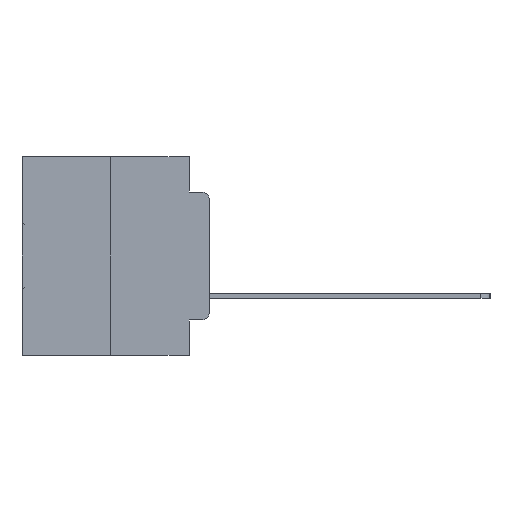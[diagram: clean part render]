
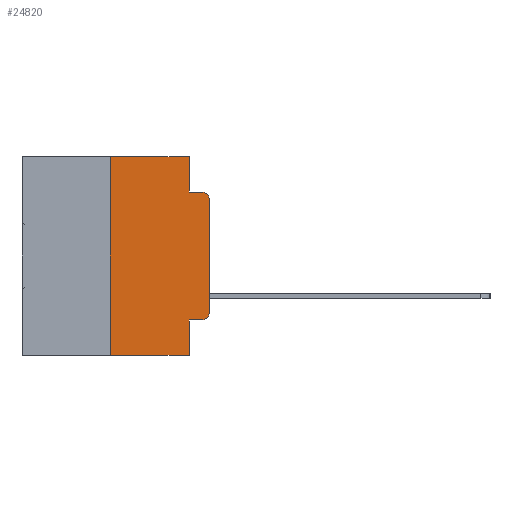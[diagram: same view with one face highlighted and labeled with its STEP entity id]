
A CAD part, left-side view. The second image highlights one B-rep face of the part: STEP entity #24820.
In plain terms, the highlighted planar face has unit normal (-1, 0, 0).
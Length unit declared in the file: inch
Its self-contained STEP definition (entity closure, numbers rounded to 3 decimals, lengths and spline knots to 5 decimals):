
#988 = VERTEX_POINT ( 'NONE', #23663 ) ;
#1040 = CARTESIAN_POINT ( 'NONE',  ( 0., 0.02, -0.3915 ) ) ;
#1591 = EDGE_CURVE ( 'NONE', #27273, #22141, #10794, .T. ) ;
#3335 = CARTESIAN_POINT ( 'NONE',  ( 0., 0., 0. ) ) ;
#3458 = ORIENTED_EDGE ( 'NONE', *, *, #25000, .T. ) ;
#3571 = DIRECTION ( 'NONE',  ( 0., 0., -1. ) ) ;
#3764 = VERTEX_POINT ( 'NONE', #28534 ) ;
#4169 = DIRECTION ( 'NONE',  ( 0., 0., 1. ) ) ;
#4621 = VERTEX_POINT ( 'NONE', #22576 ) ;
#4891 = AXIS2_PLACEMENT_3D ( 'NONE', #10089, #24775, #10200 ) ;
#5931 = LINE ( 'NONE', #25478, #31104 ) ;
#6651 = CARTESIAN_POINT ( 'NONE',  ( 0., 0.02, -0.1085 ) ) ;
#6950 = CARTESIAN_POINT ( 'NONE',  ( 0., 0.051, -0.4115 ) ) ;
#6999 = ORIENTED_EDGE ( 'NONE', *, *, #1591, .F. ) ;
#7049 = FACE_OUTER_BOUND ( 'NONE', #20201, .T. ) ;
#7305 = CARTESIAN_POINT ( 'NONE',  ( 0., 0.051, 0. ) ) ;
#7730 = PLANE ( 'NONE',  #4891 ) ;
#8186 = ORIENTED_EDGE ( 'NONE', *, *, #10568, .F. ) ;
#8325 = CARTESIAN_POINT ( 'NONE',  ( 0., 0.051, -0.4115 ) ) ;
#8452 = DIRECTION ( 'NONE',  ( 0., -1., 0. ) ) ;
#9172 = DIRECTION ( 'NONE',  ( 0., 0., -1. ) ) ;
#9244 = AXIS2_PLACEMENT_3D ( 'NONE', #1040, #18302, #3571 ) ;
#10089 = CARTESIAN_POINT ( 'NONE',  ( 0., 0.473, 0. ) ) ;
#10200 = DIRECTION ( 'NONE',  ( 0., 0., -1. ) ) ;
#10288 = VERTEX_POINT ( 'NONE', #20030 ) ;
#10474 = EDGE_CURVE ( 'NONE', #10288, #25255, #24350, .T. ) ;
#10568 = EDGE_CURVE ( 'NONE', #11754, #3764, #27742, .T. ) ;
#10794 = LINE ( 'NONE', #30695, #17292 ) ;
#11110 = EDGE_CURVE ( 'NONE', #22141, #13493, #5931, .T. ) ;
#11323 = EDGE_CURVE ( 'NONE', #20082, #27273, #25884, .T. ) ;
#11754 = VERTEX_POINT ( 'NONE', #8325 ) ;
#11922 = CARTESIAN_POINT ( 'NONE',  ( 0., 0.473, -0.5 ) ) ;
#12048 = EDGE_CURVE ( 'NONE', #4621, #3764, #23223, .T. ) ;
#12627 = CARTESIAN_POINT ( 'NONE',  ( 0., 0.051, -0.0885 ) ) ;
#13260 = DIRECTION ( 'NONE',  ( 0., 0., 1. ) ) ;
#13493 = VERTEX_POINT ( 'NONE', #22747 ) ;
#13698 = CARTESIAN_POINT ( 'NONE',  ( 0., 0.051, 0. ) ) ;
#13755 = EDGE_CURVE ( 'NONE', #4621, #20082, #24603, .T. ) ;
#14351 = DIRECTION ( 'NONE',  ( 0., -1., 0. ) ) ;
#14838 = VECTOR ( 'NONE', #25820, 39.37008 ) ;
#15492 = VECTOR ( 'NONE', #13260, 39.37008 ) ;
#16269 = LINE ( 'NONE', #3335, #15492 ) ;
#16579 = CARTESIAN_POINT ( 'NONE',  ( 0., 0.473, 0. ) ) ;
#17292 = VECTOR ( 'NONE', #28388, 39.37008 ) ;
#17509 = VECTOR ( 'NONE', #28945, 39.37008 ) ;
#17864 = VECTOR ( 'NONE', #14351, 39.37008 ) ;
#18302 = DIRECTION ( 'NONE',  ( -1., 0., 0. ) ) ;
#18519 = ORIENTED_EDGE ( 'NONE', *, *, #10474, .T. ) ;
#19002 = DIRECTION ( 'NONE',  ( 0., -1., 0. ) ) ;
#19450 = VECTOR ( 'NONE', #19002, 39.37008 ) ;
#19624 = ORIENTED_EDGE ( 'NONE', *, *, #27128, .T. ) ;
#19652 = ORIENTED_EDGE ( 'NONE', *, *, #12048, .T. ) ;
#20030 = CARTESIAN_POINT ( 'NONE',  ( 0., 0.02, -0.4115 ) ) ;
#20082 = VERTEX_POINT ( 'NONE', #21308 ) ;
#20161 = EDGE_CURVE ( 'NONE', #11754, #10288, #31493, .T. ) ;
#20201 = EDGE_LOOP ( 'NONE', ( #3458, #19624, #22685, #6999, #27213, #28751, #19652, #8186, #22718, #18519 ) ) ;
#21308 = CARTESIAN_POINT ( 'NONE',  ( 0., 0.25, 0. ) ) ;
#21500 = CIRCLE ( 'NONE', #28917, 0.02 ) ;
#22141 = VERTEX_POINT ( 'NONE', #12627 ) ;
#22576 = CARTESIAN_POINT ( 'NONE',  ( 0., 0.25, -0.5 ) ) ;
#22685 = ORIENTED_EDGE ( 'NONE', *, *, #11110, .F. ) ;
#22718 = ORIENTED_EDGE ( 'NONE', *, *, #20161, .T. ) ;
#22747 = CARTESIAN_POINT ( 'NONE',  ( 0., 0.02, -0.0885 ) ) ;
#23223 = LINE ( 'NONE', #11922, #17509 ) ;
#23663 = CARTESIAN_POINT ( 'NONE',  ( 0., 0., -0.1085 ) ) ;
#23750 = DIRECTION ( 'NONE',  ( -1., 0., 0. ) ) ;
#23844 = VECTOR ( 'NONE', #4169, 39.37008 ) ;
#24350 = CIRCLE ( 'NONE', #9244, 0.02 ) ;
#24603 = LINE ( 'NONE', #26187, #23844 ) ;
#24775 = DIRECTION ( 'NONE',  ( 1., 0., 0. ) ) ;
#24820 = ADVANCED_FACE ( 'NONE', ( #7049 ), #7730, .F. ) ;
#25000 = EDGE_CURVE ( 'NONE', #25255, #988, #16269, .T. ) ;
#25255 = VERTEX_POINT ( 'NONE', #26862 ) ;
#25478 = CARTESIAN_POINT ( 'NONE',  ( 0., 0.051, -0.0885 ) ) ;
#25820 = DIRECTION ( 'NONE',  ( 0., 0., -1. ) ) ;
#25884 = LINE ( 'NONE', #16579, #19450 ) ;
#26187 = CARTESIAN_POINT ( 'NONE',  ( 0., 0.25, 0. ) ) ;
#26862 = CARTESIAN_POINT ( 'NONE',  ( 0., 0., -0.3915 ) ) ;
#27128 = EDGE_CURVE ( 'NONE', #988, #13493, #21500, .T. ) ;
#27213 = ORIENTED_EDGE ( 'NONE', *, *, #11323, .F. ) ;
#27273 = VERTEX_POINT ( 'NONE', #7305 ) ;
#27742 = LINE ( 'NONE', #13698, #14838 ) ;
#28388 = DIRECTION ( 'NONE',  ( 0., 0., -1. ) ) ;
#28534 = CARTESIAN_POINT ( 'NONE',  ( 0., 0.051, -0.5 ) ) ;
#28751 = ORIENTED_EDGE ( 'NONE', *, *, #13755, .F. ) ;
#28917 = AXIS2_PLACEMENT_3D ( 'NONE', #6651, #23750, #9172 ) ;
#28945 = DIRECTION ( 'NONE',  ( 0., -1., 0. ) ) ;
#30695 = CARTESIAN_POINT ( 'NONE',  ( 0., 0.051, 0. ) ) ;
#31104 = VECTOR ( 'NONE', #8452, 39.37008 ) ;
#31493 = LINE ( 'NONE', #6950, #17864 ) ;
